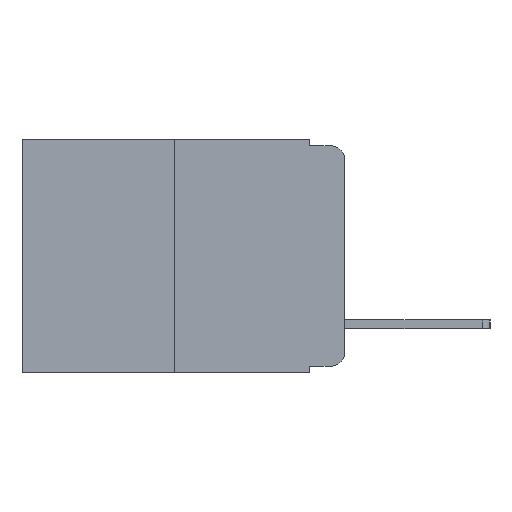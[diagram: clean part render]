
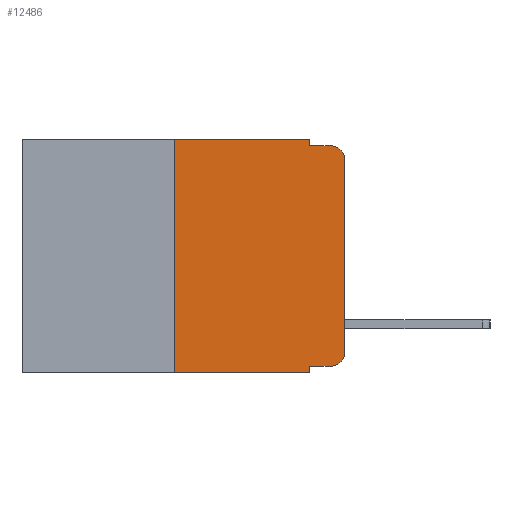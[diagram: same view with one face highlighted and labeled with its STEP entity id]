
A CAD part, left-side view. The second image highlights one B-rep face of the part: STEP entity #12486.
In plain terms, the highlighted planar face has unit normal (-1, 0, 0).
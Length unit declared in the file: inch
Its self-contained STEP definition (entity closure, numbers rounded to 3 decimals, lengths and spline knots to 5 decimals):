
#364 = CARTESIAN_POINT ( 'NONE',  ( 0., 0., 0. ) ) ;
#513 = CARTESIAN_POINT ( 'NONE',  ( 0., 0.02, -0.333 ) ) ;
#596 = EDGE_CURVE ( 'NONE', #3165, #7175, #3952, .T. ) ;
#1339 = VECTOR ( 'NONE', #6920, 39.37008 ) ;
#1458 = CARTESIAN_POINT ( 'NONE',  ( 0., 0.051, -0.01 ) ) ;
#1704 = CARTESIAN_POINT ( 'NONE',  ( 0., 0.02, -0.313 ) ) ;
#1875 = ORIENTED_EDGE ( 'NONE', *, *, #1932, .T. ) ;
#1932 = EDGE_CURVE ( 'NONE', #22323, #7175, #22299, .T. ) ;
#3164 = LINE ( 'NONE', #14400, #12724 ) ;
#3165 = VERTEX_POINT ( 'NONE', #22052 ) ;
#3230 = DIRECTION ( 'NONE',  ( 0., -1., 0. ) ) ;
#3236 = CARTESIAN_POINT ( 'NONE',  ( 0., 0.051, -0.333 ) ) ;
#3259 = EDGE_CURVE ( 'NONE', #7917, #22323, #15363, .T. ) ;
#3435 = ORIENTED_EDGE ( 'NONE', *, *, #596, .F. ) ;
#3453 = DIRECTION ( 'NONE',  ( 0., -1., 0. ) ) ;
#3662 = DIRECTION ( 'NONE',  ( 0., 0., -1. ) ) ;
#3952 = LINE ( 'NONE', #1458, #18088 ) ;
#4076 = VECTOR ( 'NONE', #21936, 39.37008 ) ;
#4328 = CARTESIAN_POINT ( 'NONE',  ( 0., 0., -0.03 ) ) ;
#4614 = LINE ( 'NONE', #19080, #23202 ) ;
#5585 = ORIENTED_EDGE ( 'NONE', *, *, #19670, .T. ) ;
#5662 = FACE_OUTER_BOUND ( 'NONE', #8342, .T. ) ;
#5699 = AXIS2_PLACEMENT_3D ( 'NONE', #1704, #14951, #3662 ) ;
#5859 = DIRECTION ( 'NONE',  ( 0., 0., -1. ) ) ;
#5873 = ORIENTED_EDGE ( 'NONE', *, *, #3259, .T. ) ;
#6078 = VERTEX_POINT ( 'NONE', #9928 ) ;
#6180 = CARTESIAN_POINT ( 'NONE',  ( 0., 0.02, -0.03 ) ) ;
#6292 = EDGE_CURVE ( 'NONE', #23592, #12553, #11597, .T. ) ;
#6337 = CIRCLE ( 'NONE', #5699, 0.02 ) ;
#6673 = CARTESIAN_POINT ( 'NONE',  ( 0., 0.473, 0. ) ) ;
#6920 = DIRECTION ( 'NONE',  ( 0., -1., 0. ) ) ;
#7175 = VERTEX_POINT ( 'NONE', #8973 ) ;
#7917 = VERTEX_POINT ( 'NONE', #8469 ) ;
#8149 = DIRECTION ( 'NONE',  ( 0., 0., -1. ) ) ;
#8338 = ORIENTED_EDGE ( 'NONE', *, *, #6292, .F. ) ;
#8342 = EDGE_LOOP ( 'NONE', ( #5873, #1875, #3435, #16782, #8338, #13254, #22982, #18937, #5585, #20005 ) ) ;
#8469 = CARTESIAN_POINT ( 'NONE',  ( 0., 0., -0.313 ) ) ;
#8973 = CARTESIAN_POINT ( 'NONE',  ( 0., 0.02, -0.01 ) ) ;
#8979 = CARTESIAN_POINT ( 'NONE',  ( 0., 0.051, 0. ) ) ;
#8993 = DIRECTION ( 'NONE',  ( 0., 0., 1. ) ) ;
#9305 = LINE ( 'NONE', #16765, #4076 ) ;
#9531 = VECTOR ( 'NONE', #5859, 39.37008 ) ;
#9928 = CARTESIAN_POINT ( 'NONE',  ( 0., 0.25, -0.343 ) ) ;
#10073 = VERTEX_POINT ( 'NONE', #3236 ) ;
#10166 = VERTEX_POINT ( 'NONE', #19866 ) ;
#10456 = PLANE ( 'NONE',  #10725 ) ;
#10672 = VERTEX_POINT ( 'NONE', #513 ) ;
#10725 = AXIS2_PLACEMENT_3D ( 'NONE', #6673, #22722, #12305 ) ;
#10840 = AXIS2_PLACEMENT_3D ( 'NONE', #6180, #18843, #8149 ) ;
#11597 = LINE ( 'NONE', #19472, #1339 ) ;
#12305 = DIRECTION ( 'NONE',  ( 0., 0., -1. ) ) ;
#12486 = ADVANCED_FACE ( 'NONE', ( #5662 ), #10456, .F. ) ;
#12553 = VERTEX_POINT ( 'NONE', #8979 ) ;
#12724 = VECTOR ( 'NONE', #8993, 39.37008 ) ;
#13254 = ORIENTED_EDGE ( 'NONE', *, *, #21973, .F. ) ;
#14206 = CARTESIAN_POINT ( 'NONE',  ( 0., 0.25, 0. ) ) ;
#14368 = LINE ( 'NONE', #16850, #9531 ) ;
#14400 = CARTESIAN_POINT ( 'NONE',  ( 0., 0.25, 0. ) ) ;
#14951 = DIRECTION ( 'NONE',  ( -1., 0., 0. ) ) ;
#15363 = LINE ( 'NONE', #364, #23436 ) ;
#15514 = DIRECTION ( 'NONE',  ( 0., 0., 1. ) ) ;
#16765 = CARTESIAN_POINT ( 'NONE',  ( 0., 0.051, 0. ) ) ;
#16782 = ORIENTED_EDGE ( 'NONE', *, *, #23138, .F. ) ;
#16850 = CARTESIAN_POINT ( 'NONE',  ( 0., 0.051, 0. ) ) ;
#18088 = VECTOR ( 'NONE', #3453, 39.37008 ) ;
#18534 = EDGE_CURVE ( 'NONE', #10672, #7917, #6337, .T. ) ;
#18843 = DIRECTION ( 'NONE',  ( -1., 0., 0. ) ) ;
#18937 = ORIENTED_EDGE ( 'NONE', *, *, #20796, .F. ) ;
#19080 = CARTESIAN_POINT ( 'NONE',  ( 0., 0.473, -0.343 ) ) ;
#19472 = CARTESIAN_POINT ( 'NONE',  ( 0., 0.473, 0. ) ) ;
#19670 = EDGE_CURVE ( 'NONE', #10073, #10672, #21681, .T. ) ;
#19866 = CARTESIAN_POINT ( 'NONE',  ( 0., 0.051, -0.343 ) ) ;
#20005 = ORIENTED_EDGE ( 'NONE', *, *, #18534, .T. ) ;
#20786 = DIRECTION ( 'NONE',  ( 0., -1., 0. ) ) ;
#20796 = EDGE_CURVE ( 'NONE', #10073, #10166, #9305, .T. ) ;
#21152 = VECTOR ( 'NONE', #3230, 39.37008 ) ;
#21361 = CARTESIAN_POINT ( 'NONE',  ( 0., 0.051, -0.333 ) ) ;
#21681 = LINE ( 'NONE', #21361, #21152 ) ;
#21936 = DIRECTION ( 'NONE',  ( 0., 0., -1. ) ) ;
#21973 = EDGE_CURVE ( 'NONE', #6078, #23592, #3164, .T. ) ;
#22052 = CARTESIAN_POINT ( 'NONE',  ( 0., 0.051, -0.01 ) ) ;
#22299 = CIRCLE ( 'NONE', #10840, 0.02 ) ;
#22323 = VERTEX_POINT ( 'NONE', #4328 ) ;
#22722 = DIRECTION ( 'NONE',  ( 1., 0., 0. ) ) ;
#22982 = ORIENTED_EDGE ( 'NONE', *, *, #23427, .T. ) ;
#23138 = EDGE_CURVE ( 'NONE', #12553, #3165, #14368, .T. ) ;
#23202 = VECTOR ( 'NONE', #20786, 39.37008 ) ;
#23427 = EDGE_CURVE ( 'NONE', #6078, #10166, #4614, .T. ) ;
#23436 = VECTOR ( 'NONE', #15514, 39.37008 ) ;
#23592 = VERTEX_POINT ( 'NONE', #14206 ) ;
